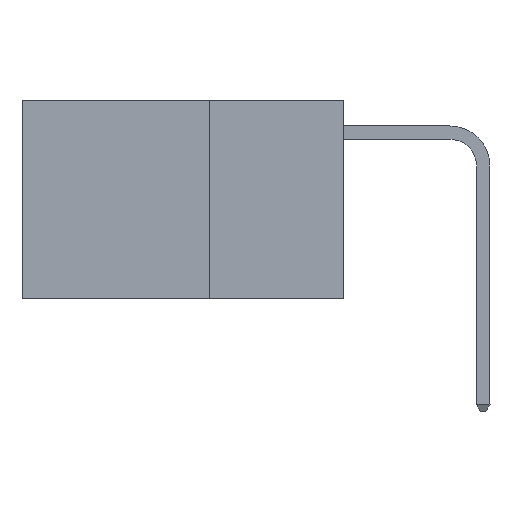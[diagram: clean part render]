
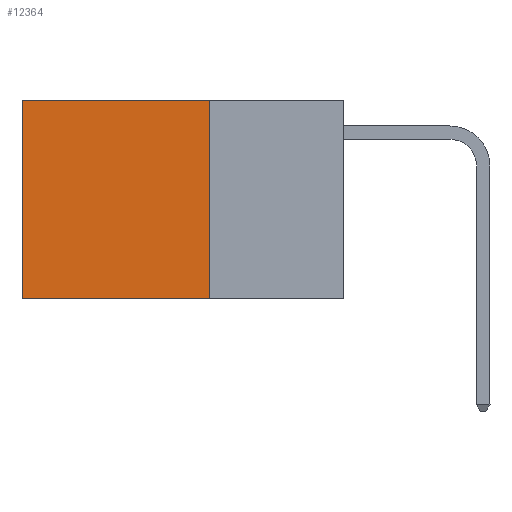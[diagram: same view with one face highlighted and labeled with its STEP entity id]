
A CAD part, left-side view. The second image highlights one B-rep face of the part: STEP entity #12364.
In plain terms, the highlighted planar face has unit normal (-1, 0, 0).
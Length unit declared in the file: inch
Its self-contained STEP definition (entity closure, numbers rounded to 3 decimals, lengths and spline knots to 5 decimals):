
#108 = CARTESIAN_POINT ( 'NONE',  ( 0.2625, 0.6, 0. ) ) ;
#124 = VERTEX_POINT ( 'NONE', #10820 ) ;
#310 = EDGE_CURVE ( 'NONE', #124, #7692, #2889, .T. ) ;
#720 = VECTOR ( 'NONE', #8954, 39.37008 ) ;
#744 = CARTESIAN_POINT ( 'NONE',  ( 0.2625, 0.25, 0. ) ) ;
#1489 = PLANE ( 'NONE',  #8833 ) ;
#1676 = CARTESIAN_POINT ( 'NONE',  ( 0.2625, 0.6, 0. ) ) ;
#2036 = LINE ( 'NONE', #744, #11358 ) ;
#2042 = DIRECTION ( 'NONE',  ( 0., 1., 0. ) ) ;
#2074 = LINE ( 'NONE', #2124, #14537 ) ;
#2124 = CARTESIAN_POINT ( 'NONE',  ( 0.2625, 0.25, -0.37 ) ) ;
#2343 = CARTESIAN_POINT ( 'NONE',  ( 0.2625, 0.6, -0.37 ) ) ;
#2545 = CARTESIAN_POINT ( 'NONE',  ( 0.2625, 0.25, -0.37 ) ) ;
#2718 = DIRECTION ( 'NONE',  ( 0., 0., -1. ) ) ;
#2834 = EDGE_CURVE ( 'NONE', #7692, #4462, #2074, .T. ) ;
#2889 = LINE ( 'NONE', #13218, #15304 ) ;
#3592 = LINE ( 'NONE', #1676, #720 ) ;
#3876 = CARTESIAN_POINT ( 'NONE',  ( 0.2625, 0.25, 0. ) ) ;
#4260 = EDGE_CURVE ( 'NONE', #124, #14256, #2036, .T. ) ;
#4333 = ORIENTED_EDGE ( 'NONE', *, *, #310, .F. ) ;
#4426 = FACE_OUTER_BOUND ( 'NONE', #4436, .T. ) ;
#4436 = EDGE_LOOP ( 'NONE', ( #13236, #8096, #4333, #11419 ) ) ;
#4462 = VERTEX_POINT ( 'NONE', #2343 ) ;
#7692 = VERTEX_POINT ( 'NONE', #2545 ) ;
#8096 = ORIENTED_EDGE ( 'NONE', *, *, #2834, .F. ) ;
#8833 = AXIS2_PLACEMENT_3D ( 'NONE', #3876, #10018, #2718 ) ;
#8954 = DIRECTION ( 'NONE',  ( 0., 0., -1. ) ) ;
#9571 = EDGE_CURVE ( 'NONE', #14256, #4462, #3592, .T. ) ;
#10018 = DIRECTION ( 'NONE',  ( 1., 0., 0. ) ) ;
#10820 = CARTESIAN_POINT ( 'NONE',  ( 0.2625, 0.25, 0. ) ) ;
#11358 = VECTOR ( 'NONE', #11622, 39.37008 ) ;
#11419 = ORIENTED_EDGE ( 'NONE', *, *, #4260, .T. ) ;
#11622 = DIRECTION ( 'NONE',  ( 0., 1., 0. ) ) ;
#12364 = ADVANCED_FACE ( 'NONE', ( #4426 ), #1489, .F. ) ;
#12987 = DIRECTION ( 'NONE',  ( 0., 0., -1. ) ) ;
#13218 = CARTESIAN_POINT ( 'NONE',  ( 0.2625, 0.25, 0. ) ) ;
#13236 = ORIENTED_EDGE ( 'NONE', *, *, #9571, .T. ) ;
#14256 = VERTEX_POINT ( 'NONE', #108 ) ;
#14537 = VECTOR ( 'NONE', #2042, 39.37008 ) ;
#15304 = VECTOR ( 'NONE', #12987, 39.37008 ) ;
